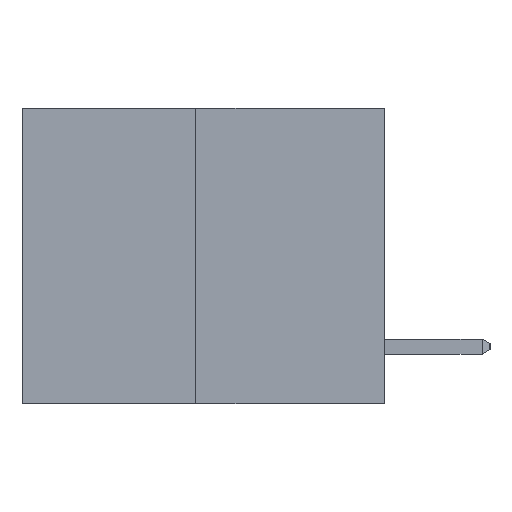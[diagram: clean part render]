
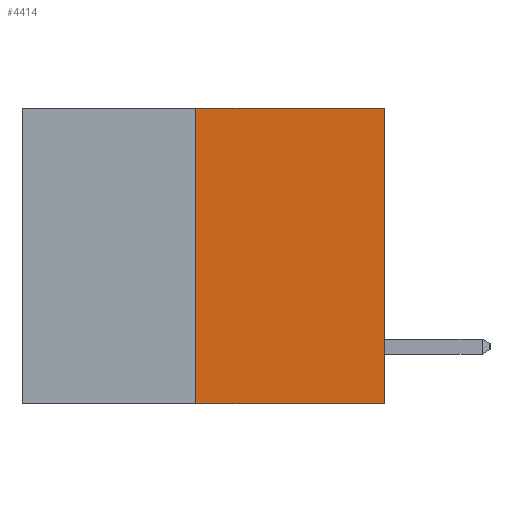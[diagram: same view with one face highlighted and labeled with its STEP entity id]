
A CAD part, left-side view. The second image highlights one B-rep face of the part: STEP entity #4414.
In plain terms, the highlighted planar face has unit normal (-1, 0, 0).
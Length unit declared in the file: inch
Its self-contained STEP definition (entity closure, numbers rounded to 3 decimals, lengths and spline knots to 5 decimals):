
#12 = ORIENTED_EDGE ( 'NONE', *, *, #3056, .T. ) ;
#606 = CARTESIAN_POINT ( 'NONE',  ( 0., 0.6, 0. ) ) ;
#1191 = EDGE_CURVE ( 'NONE', #13445, #14602, #14485, .T. ) ;
#1771 = AXIS2_PLACEMENT_3D ( 'NONE', #7754, #10135, #2881 ) ;
#2329 = CARTESIAN_POINT ( 'NONE',  ( 0., 0., 0. ) ) ;
#2881 = DIRECTION ( 'NONE',  ( 0., 0., -1. ) ) ;
#3056 = EDGE_CURVE ( 'NONE', #10282, #14602, #3447, .T. ) ;
#3447 = LINE ( 'NONE', #2329, #12538 ) ;
#3691 = CARTESIAN_POINT ( 'NONE',  ( 0., 0., -0.49 ) ) ;
#4414 = ADVANCED_FACE ( 'NONE', ( #9349 ), #14818, .F. ) ;
#4456 = EDGE_LOOP ( 'NONE', ( #7093, #13024, #12, #6929 ) ) ;
#5724 = LINE ( 'NONE', #10782, #14763 ) ;
#6231 = DIRECTION ( 'NONE',  ( 0., -1., 0. ) ) ;
#6929 = ORIENTED_EDGE ( 'NONE', *, *, #1191, .F. ) ;
#6994 = DIRECTION ( 'NONE',  ( 0., -1., 0. ) ) ;
#7032 = LINE ( 'NONE', #7688, #12203 ) ;
#7093 = ORIENTED_EDGE ( 'NONE', *, *, #8991, .F. ) ;
#7650 = CARTESIAN_POINT ( 'NONE',  ( 0., 0., 0. ) ) ;
#7688 = CARTESIAN_POINT ( 'NONE',  ( 0., 0.312, -0.49 ) ) ;
#7746 = DIRECTION ( 'NONE',  ( 0., 0., 1. ) ) ;
#7754 = CARTESIAN_POINT ( 'NONE',  ( 0., 0.6, 0. ) ) ;
#7841 = VECTOR ( 'NONE', #6994, 39.37008 ) ;
#8284 = CARTESIAN_POINT ( 'NONE',  ( 0., 0.312, -0.49 ) ) ;
#8368 = VERTEX_POINT ( 'NONE', #8284 ) ;
#8991 = EDGE_CURVE ( 'NONE', #8368, #13445, #7032, .T. ) ;
#9272 = EDGE_CURVE ( 'NONE', #8368, #10282, #5724, .T. ) ;
#9349 = FACE_OUTER_BOUND ( 'NONE', #4456, .T. ) ;
#9446 = DIRECTION ( 'NONE',  ( 0., 0., 1. ) ) ;
#10135 = DIRECTION ( 'NONE',  ( 1., 0., 0. ) ) ;
#10282 = VERTEX_POINT ( 'NONE', #3691 ) ;
#10782 = CARTESIAN_POINT ( 'NONE',  ( 0., 0.6, -0.49 ) ) ;
#12203 = VECTOR ( 'NONE', #7746, 39.37008 ) ;
#12538 = VECTOR ( 'NONE', #9446, 39.37008 ) ;
#13024 = ORIENTED_EDGE ( 'NONE', *, *, #9272, .T. ) ;
#13445 = VERTEX_POINT ( 'NONE', #13790 ) ;
#13790 = CARTESIAN_POINT ( 'NONE',  ( 0., 0.312, 0. ) ) ;
#14485 = LINE ( 'NONE', #606, #7841 ) ;
#14602 = VERTEX_POINT ( 'NONE', #7650 ) ;
#14763 = VECTOR ( 'NONE', #6231, 39.37008 ) ;
#14818 = PLANE ( 'NONE',  #1771 ) ;
